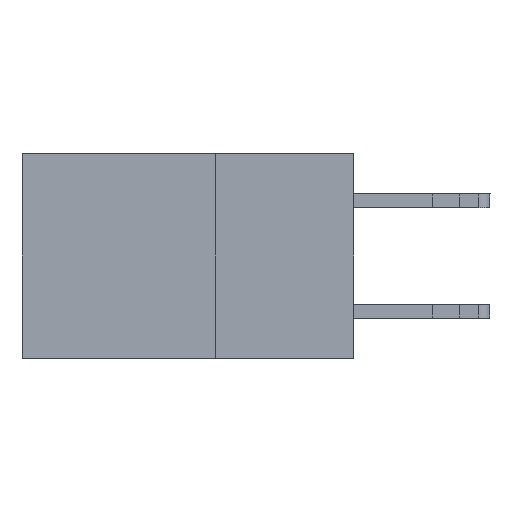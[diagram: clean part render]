
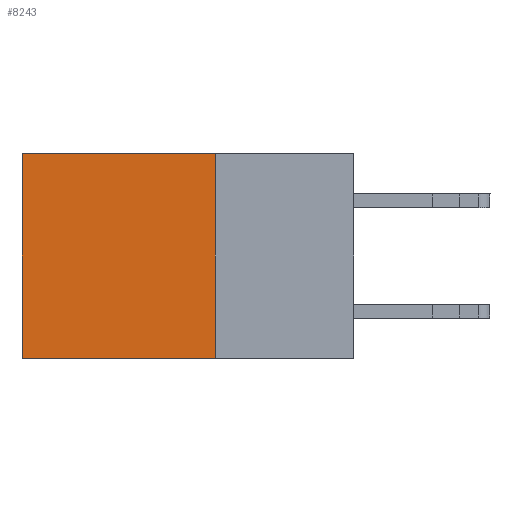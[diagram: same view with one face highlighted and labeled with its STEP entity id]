
A CAD part, left-side view. The second image highlights one B-rep face of the part: STEP entity #8243.
In plain terms, the highlighted planar face has unit normal (-1, 0, 0).
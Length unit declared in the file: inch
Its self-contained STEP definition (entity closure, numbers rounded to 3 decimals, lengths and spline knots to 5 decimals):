
#348 = VERTEX_POINT ( 'NONE', #7179 ) ;
#997 = EDGE_CURVE ( 'NONE', #16640, #10997, #2852, .T. ) ;
#1244 = DIRECTION ( 'NONE',  ( 1., 0., 0. ) ) ;
#1658 = EDGE_CURVE ( 'NONE', #12315, #348, #16020, .T. ) ;
#2680 = LINE ( 'NONE', #18477, #10665 ) ;
#2852 = LINE ( 'NONE', #16605, #25326 ) ;
#3402 = ORIENTED_EDGE ( 'NONE', *, *, #4117, .F. ) ;
#4117 = EDGE_CURVE ( 'NONE', #348, #10997, #2680, .T. ) ;
#4671 = CARTESIAN_POINT ( 'NONE',  ( 0.2875, 0.6, -0.37 ) ) ;
#4675 = FACE_OUTER_BOUND ( 'NONE', #6271, .T. ) ;
#5974 = CARTESIAN_POINT ( 'NONE',  ( 0.2875, 0.25, 0. ) ) ;
#6271 = EDGE_LOOP ( 'NONE', ( #18409, #3402, #19728, #10172 ) ) ;
#6654 = DIRECTION ( 'NONE',  ( 0., 1., 0. ) ) ;
#6749 = LINE ( 'NONE', #16280, #17938 ) ;
#7089 = AXIS2_PLACEMENT_3D ( 'NONE', #11336, #1244, #21179 ) ;
#7179 = CARTESIAN_POINT ( 'NONE',  ( 0.2875, 0.25, -0.37 ) ) ;
#8243 = ADVANCED_FACE ( 'NONE', ( #4675 ), #12640, .F. ) ;
#10172 = ORIENTED_EDGE ( 'NONE', *, *, #21984, .T. ) ;
#10665 = VECTOR ( 'NONE', #6654, 39.37008 ) ;
#10997 = VERTEX_POINT ( 'NONE', #4671 ) ;
#11336 = CARTESIAN_POINT ( 'NONE',  ( 0.2875, 0.25, 0. ) ) ;
#12315 = VERTEX_POINT ( 'NONE', #17318 ) ;
#12640 = PLANE ( 'NONE',  #7089 ) ;
#16020 = LINE ( 'NONE', #5974, #16633 ) ;
#16280 = CARTESIAN_POINT ( 'NONE',  ( 0.2875, 0.25, 0. ) ) ;
#16605 = CARTESIAN_POINT ( 'NONE',  ( 0.2875, 0.6, 0. ) ) ;
#16633 = VECTOR ( 'NONE', #18056, 39.37008 ) ;
#16640 = VERTEX_POINT ( 'NONE', #17081 ) ;
#17081 = CARTESIAN_POINT ( 'NONE',  ( 0.2875, 0.6, 0. ) ) ;
#17318 = CARTESIAN_POINT ( 'NONE',  ( 0.2875, 0.25, 0. ) ) ;
#17938 = VECTOR ( 'NONE', #18441, 39.37008 ) ;
#18056 = DIRECTION ( 'NONE',  ( 0., 0., -1. ) ) ;
#18409 = ORIENTED_EDGE ( 'NONE', *, *, #997, .T. ) ;
#18441 = DIRECTION ( 'NONE',  ( 0., 1., 0. ) ) ;
#18477 = CARTESIAN_POINT ( 'NONE',  ( 0.2875, 0.25, -0.37 ) ) ;
#18783 = DIRECTION ( 'NONE',  ( 0., 0., -1. ) ) ;
#19728 = ORIENTED_EDGE ( 'NONE', *, *, #1658, .F. ) ;
#21179 = DIRECTION ( 'NONE',  ( 0., 0., -1. ) ) ;
#21984 = EDGE_CURVE ( 'NONE', #12315, #16640, #6749, .T. ) ;
#25326 = VECTOR ( 'NONE', #18783, 39.37008 ) ;
